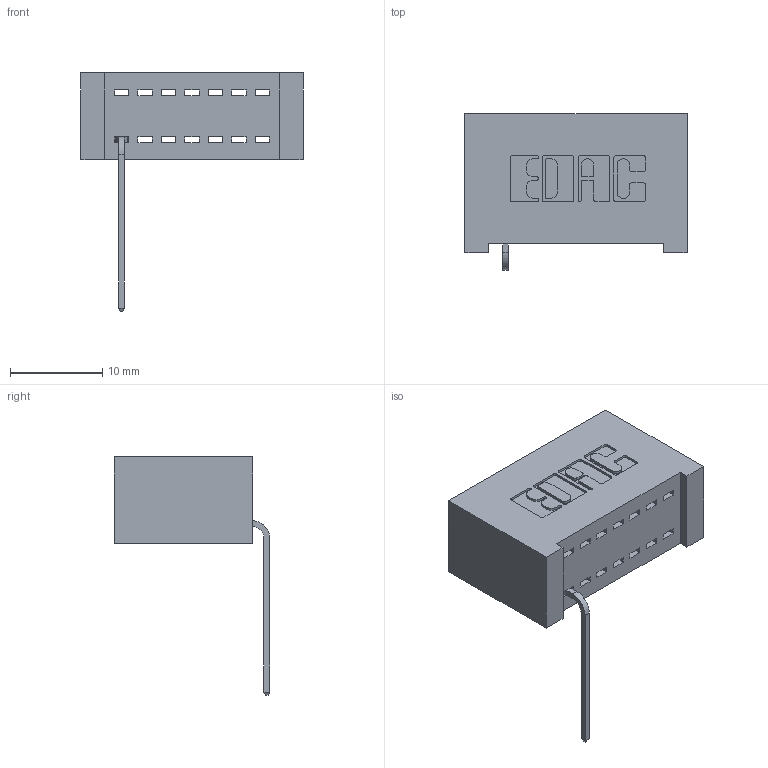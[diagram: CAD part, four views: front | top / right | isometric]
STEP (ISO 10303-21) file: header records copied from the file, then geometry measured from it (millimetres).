
FILE_DESCRIPTION (( 'STEP AP203' ), '1' );
FILE_NAME ('392-007-559-101.STEP', '2018-08-14T19:03:47', ( '' ), ( '' ), 'SwSTEP 2.0', 'SolidWorks 2016', '' );
FILE_SCHEMA (( 'CONFIG_CONTROL_DESIGN' ));
Length unit declared in the file: inch
Products named in the file (3): 342 Part_Lugless; 345-292-001_558 559 Tail - 1; 392-007-559-101
Assembly tree (2 placements, depth 2):
  392-007-559-101
    342 Part_Lugless
    345-292-001_558 559 Tail - 1
Bounding box: 24.03 x 16.83 x 25.78 mm (x, y, z)
Volume: 2321.6 mm3; surface area: 2742.3 mm2
Topology: 2 solids, 2 shells, 234 faces, 709 edges, 470 vertices
Faces by surface type: plane 178, cylinder 56
Entity records: 8289 total; most frequent: CARTESIAN_POINT 1469, ORIENTED_EDGE 1418, DIRECTION 1295, EDGE_CURVE 709, VECTOR 589, LINE 589, VERTEX_POINT 470, AXIS2_PLACEMENT_3D 353
